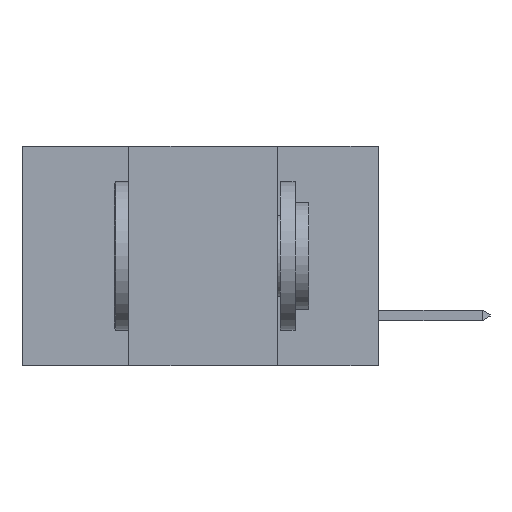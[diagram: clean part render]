
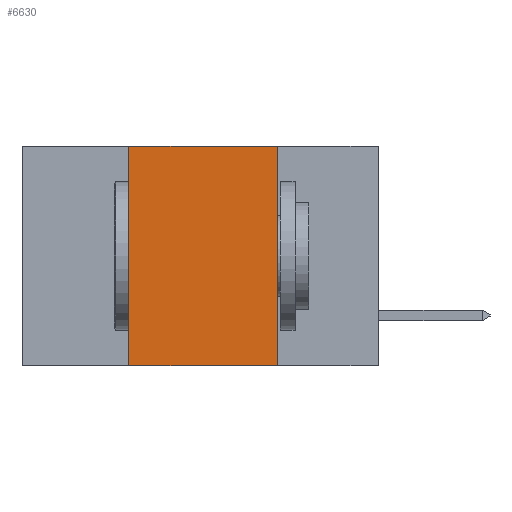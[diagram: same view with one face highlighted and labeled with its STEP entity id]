
A CAD part, left-side view. The second image highlights one B-rep face of the part: STEP entity #6630.
In plain terms, the highlighted planar face has unit normal (-1, 0, 0).
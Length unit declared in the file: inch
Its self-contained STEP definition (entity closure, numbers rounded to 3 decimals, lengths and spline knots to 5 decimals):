
#485 = DIRECTION ( 'NONE',  ( 0., 0., 1. ) ) ;
#639 = VERTEX_POINT ( 'NONE', #9963 ) ;
#642 = FACE_OUTER_BOUND ( 'NONE', #9794, .T. ) ;
#787 = ORIENTED_EDGE ( 'NONE', *, *, #3772, .F. ) ;
#948 = VERTEX_POINT ( 'NONE', #1716 ) ;
#981 = EDGE_CURVE ( 'NONE', #6245, #948, #9434, .T. ) ;
#1413 = CARTESIAN_POINT ( 'NONE',  ( 0., 0.42, -0.37 ) ) ;
#1643 = CARTESIAN_POINT ( 'NONE',  ( 0., 0.6, -0.37 ) ) ;
#1716 = CARTESIAN_POINT ( 'NONE',  ( 0., 0.42, 0. ) ) ;
#2471 = DIRECTION ( 'NONE',  ( 0., 0., -1. ) ) ;
#2517 = DIRECTION ( 'NONE',  ( 1., 0., 0. ) ) ;
#3650 = ORIENTED_EDGE ( 'NONE', *, *, #6862, .F. ) ;
#3772 = EDGE_CURVE ( 'NONE', #639, #4473, #4236, .T. ) ;
#3947 = PLANE ( 'NONE',  #9952 ) ;
#4236 = LINE ( 'NONE', #5566, #8356 ) ;
#4382 = VECTOR ( 'NONE', #6587, 39.37008 ) ;
#4473 = VERTEX_POINT ( 'NONE', #9280 ) ;
#5084 = VECTOR ( 'NONE', #485, 39.37008 ) ;
#5194 = VECTOR ( 'NONE', #5716, 39.37008 ) ;
#5449 = CARTESIAN_POINT ( 'NONE',  ( 0., 0.6, 0. ) ) ;
#5566 = CARTESIAN_POINT ( 'NONE',  ( 0., 0.17, 0. ) ) ;
#5716 = DIRECTION ( 'NONE',  ( 0., -1., 0. ) ) ;
#5891 = DIRECTION ( 'NONE',  ( 0., 0., -1. ) ) ;
#6245 = VERTEX_POINT ( 'NONE', #1413 ) ;
#6587 = DIRECTION ( 'NONE',  ( 0., -1., 0. ) ) ;
#6630 = ADVANCED_FACE ( 'NONE', ( #642 ), #3947, .F. ) ;
#6862 = EDGE_CURVE ( 'NONE', #948, #639, #9275, .T. ) ;
#7844 = EDGE_CURVE ( 'NONE', #6245, #4473, #10420, .T. ) ;
#8356 = VECTOR ( 'NONE', #5891, 39.37008 ) ;
#9275 = LINE ( 'NONE', #5449, #5194 ) ;
#9280 = CARTESIAN_POINT ( 'NONE',  ( 0., 0.17, -0.37 ) ) ;
#9430 = ORIENTED_EDGE ( 'NONE', *, *, #981, .F. ) ;
#9434 = LINE ( 'NONE', #9862, #5084 ) ;
#9652 = CARTESIAN_POINT ( 'NONE',  ( 0., 0.6, 0. ) ) ;
#9677 = ORIENTED_EDGE ( 'NONE', *, *, #7844, .T. ) ;
#9794 = EDGE_LOOP ( 'NONE', ( #787, #3650, #9430, #9677 ) ) ;
#9862 = CARTESIAN_POINT ( 'NONE',  ( 0., 0.42, 0. ) ) ;
#9952 = AXIS2_PLACEMENT_3D ( 'NONE', #9652, #2517, #2471 ) ;
#9963 = CARTESIAN_POINT ( 'NONE',  ( 0., 0.17, 0. ) ) ;
#10420 = LINE ( 'NONE', #1643, #4382 ) ;
